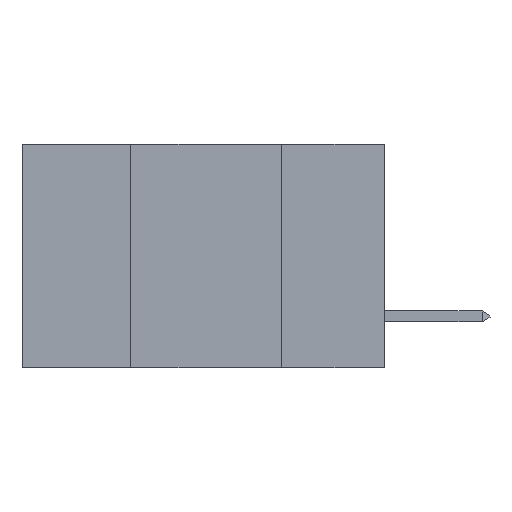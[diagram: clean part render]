
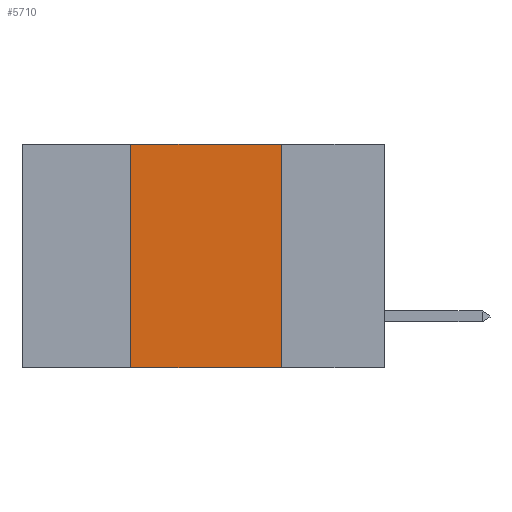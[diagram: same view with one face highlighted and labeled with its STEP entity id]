
A CAD part, left-side view. The second image highlights one B-rep face of the part: STEP entity #5710.
In plain terms, the highlighted planar face has unit normal (-1, 0, 0).
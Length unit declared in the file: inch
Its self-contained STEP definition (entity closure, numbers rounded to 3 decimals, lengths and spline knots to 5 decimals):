
#18 = VECTOR ( 'NONE', #4012, 39.37008 ) ;
#350 = DIRECTION ( 'NONE',  ( 0., -1., 0. ) ) ;
#638 = LINE ( 'NONE', #7539, #2703 ) ;
#1151 = AXIS2_PLACEMENT_3D ( 'NONE', #7506, #7966, #7489 ) ;
#1924 = CARTESIAN_POINT ( 'NONE',  ( 0., 0.6, -0.37 ) ) ;
#2050 = VERTEX_POINT ( 'NONE', #2889 ) ;
#2086 = VECTOR ( 'NONE', #9553, 39.37008 ) ;
#2443 = EDGE_CURVE ( 'NONE', #9065, #8981, #4790, .T. ) ;
#2703 = VECTOR ( 'NONE', #3709, 39.37008 ) ;
#2889 = CARTESIAN_POINT ( 'NONE',  ( 0., 0.42, 0. ) ) ;
#2985 = EDGE_CURVE ( 'NONE', #9065, #2050, #8314, .T. ) ;
#3039 = ORIENTED_EDGE ( 'NONE', *, *, #7699, .F. ) ;
#3082 = ORIENTED_EDGE ( 'NONE', *, *, #9321, .F. ) ;
#3161 = CARTESIAN_POINT ( 'NONE',  ( 0., 0.17, 0. ) ) ;
#3166 = ORIENTED_EDGE ( 'NONE', *, *, #2985, .F. ) ;
#3191 = ORIENTED_EDGE ( 'NONE', *, *, #2443, .T. ) ;
#3709 = DIRECTION ( 'NONE',  ( 0., -1., 0. ) ) ;
#4012 = DIRECTION ( 'NONE',  ( 0., 0., -1. ) ) ;
#4047 = EDGE_LOOP ( 'NONE', ( #3039, #3082, #3166, #3191 ) ) ;
#4163 = CARTESIAN_POINT ( 'NONE',  ( 0., 0.42, -0.37 ) ) ;
#4790 = LINE ( 'NONE', #1924, #8308 ) ;
#4826 = CARTESIAN_POINT ( 'NONE',  ( 0., 0.17, -0.37 ) ) ;
#5710 = ADVANCED_FACE ( 'NONE', ( #6834 ), #7497, .F. ) ;
#5831 = VERTEX_POINT ( 'NONE', #7134 ) ;
#6446 = LINE ( 'NONE', #3161, #18 ) ;
#6834 = FACE_OUTER_BOUND ( 'NONE', #4047, .T. ) ;
#7134 = CARTESIAN_POINT ( 'NONE',  ( 0., 0.17, 0. ) ) ;
#7489 = DIRECTION ( 'NONE',  ( 0., 0., -1. ) ) ;
#7497 = PLANE ( 'NONE',  #1151 ) ;
#7506 = CARTESIAN_POINT ( 'NONE',  ( 0., 0.6, 0. ) ) ;
#7539 = CARTESIAN_POINT ( 'NONE',  ( 0., 0.6, 0. ) ) ;
#7699 = EDGE_CURVE ( 'NONE', #5831, #8981, #6446, .T. ) ;
#7966 = DIRECTION ( 'NONE',  ( 1., 0., 0. ) ) ;
#8308 = VECTOR ( 'NONE', #350, 39.37008 ) ;
#8314 = LINE ( 'NONE', #9508, #2086 ) ;
#8981 = VERTEX_POINT ( 'NONE', #4826 ) ;
#9065 = VERTEX_POINT ( 'NONE', #4163 ) ;
#9321 = EDGE_CURVE ( 'NONE', #2050, #5831, #638, .T. ) ;
#9508 = CARTESIAN_POINT ( 'NONE',  ( 0., 0.42, 0. ) ) ;
#9553 = DIRECTION ( 'NONE',  ( 0., 0., 1. ) ) ;
